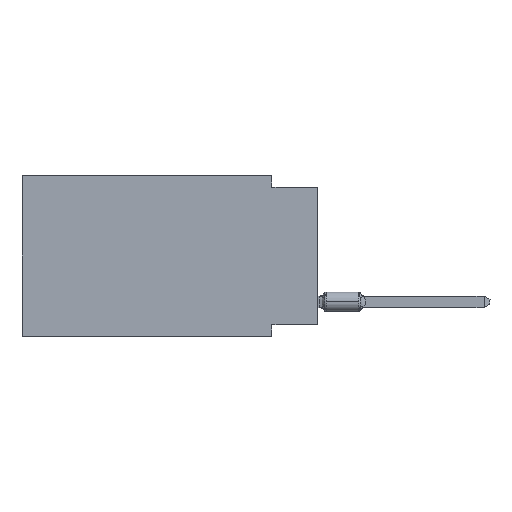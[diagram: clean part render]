
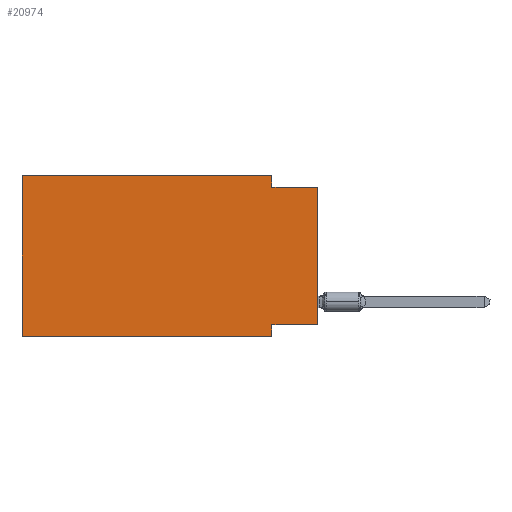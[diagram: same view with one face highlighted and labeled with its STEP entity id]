
A CAD part, left-side view. The second image highlights one B-rep face of the part: STEP entity #20974.
In plain terms, the highlighted planar face has unit normal (-1, 0, 0).
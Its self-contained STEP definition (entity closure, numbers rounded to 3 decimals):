
#352 = CARTESIAN_POINT ( 'NONE',  ( 0., 16.383, 0. ) ) ;
#388 = VERTEX_POINT ( 'NONE', #4365 ) ;
#689 = VERTEX_POINT ( 'NONE', #11810 ) ;
#819 = ORIENTED_EDGE ( 'NONE', *, *, #3849, .F. ) ;
#2015 = EDGE_CURVE ( 'NONE', #12161, #10201, #7761, .T. ) ;
#2116 = LINE ( 'NONE', #13463, #10531 ) ;
#2877 = EDGE_CURVE ( 'NONE', #23043, #689, #22561, .T. ) ;
#2887 = DIRECTION ( 'NONE',  ( 0., 0., 1. ) ) ;
#2928 = AXIS2_PLACEMENT_3D ( 'NONE', #10580, #3879, #18510 ) ;
#3102 = CARTESIAN_POINT ( 'NONE',  ( 0., 16.383, -8.89 ) ) ;
#3226 = EDGE_CURVE ( 'NONE', #19710, #15177, #5956, .T. ) ;
#3849 = EDGE_CURVE ( 'NONE', #6416, #388, #21285, .T. ) ;
#3879 = DIRECTION ( 'NONE',  ( 1., 0., 0. ) ) ;
#4365 = CARTESIAN_POINT ( 'NONE',  ( 0., 16.383, 0. ) ) ;
#4491 = EDGE_CURVE ( 'NONE', #19710, #23043, #22223, .T. ) ;
#4688 = ORIENTED_EDGE ( 'NONE', *, *, #4491, .F. ) ;
#5407 = VECTOR ( 'NONE', #5825, 1000. ) ;
#5825 = DIRECTION ( 'NONE',  ( 0., 0., -1. ) ) ;
#5866 = CARTESIAN_POINT ( 'NONE',  ( 0., 0., -8.255 ) ) ;
#5956 = LINE ( 'NONE', #11397, #23315 ) ;
#6072 = EDGE_LOOP ( 'NONE', ( #12384, #14592, #16710, #13808, #819, #9535, #22361, #4688 ) ) ;
#6402 = CARTESIAN_POINT ( 'NONE',  ( 0., 16.383, 0. ) ) ;
#6416 = VERTEX_POINT ( 'NONE', #3102 ) ;
#7072 = FACE_OUTER_BOUND ( 'NONE', #6072, .T. ) ;
#7441 = VECTOR ( 'NONE', #17009, 1000. ) ;
#7761 = LINE ( 'NONE', #11263, #5407 ) ;
#7929 = VECTOR ( 'NONE', #2887, 1000. ) ;
#8114 = CARTESIAN_POINT ( 'NONE',  ( 0., 2.54, 0. ) ) ;
#8175 = VECTOR ( 'NONE', #12751, 1000. ) ;
#8891 = PLANE ( 'NONE',  #2928 ) ;
#9360 = LINE ( 'NONE', #16605, #8175 ) ;
#9497 = DIRECTION ( 'NONE',  ( 0., -1., 0. ) ) ;
#9535 = ORIENTED_EDGE ( 'NONE', *, *, #9636, .T. ) ;
#9636 = EDGE_CURVE ( 'NONE', #6416, #689, #9360, .T. ) ;
#10201 = VERTEX_POINT ( 'NONE', #10827 ) ;
#10531 = VECTOR ( 'NONE', #9497, 1000. ) ;
#10580 = CARTESIAN_POINT ( 'NONE',  ( 0., 16.383, 0. ) ) ;
#10827 = CARTESIAN_POINT ( 'NONE',  ( 0., 2.54, -0.635 ) ) ;
#11263 = CARTESIAN_POINT ( 'NONE',  ( 0., 2.54, 0. ) ) ;
#11397 = CARTESIAN_POINT ( 'NONE',  ( 0., 0., 0. ) ) ;
#11810 = CARTESIAN_POINT ( 'NONE',  ( 0., 2.54, -8.89 ) ) ;
#12161 = VERTEX_POINT ( 'NONE', #8114 ) ;
#12384 = ORIENTED_EDGE ( 'NONE', *, *, #3226, .T. ) ;
#12751 = DIRECTION ( 'NONE',  ( 0., -1., 0. ) ) ;
#13344 = VECTOR ( 'NONE', #20512, 1000. ) ;
#13463 = CARTESIAN_POINT ( 'NONE',  ( 0., 0., -0.635 ) ) ;
#13732 = CARTESIAN_POINT ( 'NONE',  ( 0., 0., -0.635 ) ) ;
#13808 = ORIENTED_EDGE ( 'NONE', *, *, #23556, .F. ) ;
#13827 = CARTESIAN_POINT ( 'NONE',  ( 0., 2.54, -8.89 ) ) ;
#14592 = ORIENTED_EDGE ( 'NONE', *, *, #16662, .F. ) ;
#15177 = VERTEX_POINT ( 'NONE', #13732 ) ;
#15510 = DIRECTION ( 'NONE',  ( 0., 0., -1. ) ) ;
#16605 = CARTESIAN_POINT ( 'NONE',  ( 0., 16.383, -8.89 ) ) ;
#16662 = EDGE_CURVE ( 'NONE', #10201, #15177, #2116, .T. ) ;
#16710 = ORIENTED_EDGE ( 'NONE', *, *, #2015, .F. ) ;
#16790 = VECTOR ( 'NONE', #15510, 1000. ) ;
#16894 = LINE ( 'NONE', #352, #7441 ) ;
#16945 = DIRECTION ( 'NONE',  ( 0., 0., 1. ) ) ;
#17009 = DIRECTION ( 'NONE',  ( 0., -1., 0. ) ) ;
#18510 = DIRECTION ( 'NONE',  ( 0., 0., -1. ) ) ;
#19148 = CARTESIAN_POINT ( 'NONE',  ( 0., 0., -8.255 ) ) ;
#19710 = VERTEX_POINT ( 'NONE', #19148 ) ;
#19857 = CARTESIAN_POINT ( 'NONE',  ( 0., 2.54, -8.255 ) ) ;
#20512 = DIRECTION ( 'NONE',  ( 0., 1., 0. ) ) ;
#20974 = ADVANCED_FACE ( 'NONE', ( #7072 ), #8891, .F. ) ;
#21285 = LINE ( 'NONE', #6402, #7929 ) ;
#22223 = LINE ( 'NONE', #5866, #13344 ) ;
#22361 = ORIENTED_EDGE ( 'NONE', *, *, #2877, .F. ) ;
#22561 = LINE ( 'NONE', #13827, #16790 ) ;
#23043 = VERTEX_POINT ( 'NONE', #19857 ) ;
#23315 = VECTOR ( 'NONE', #16945, 1000. ) ;
#23556 = EDGE_CURVE ( 'NONE', #388, #12161, #16894, .T. ) ;
